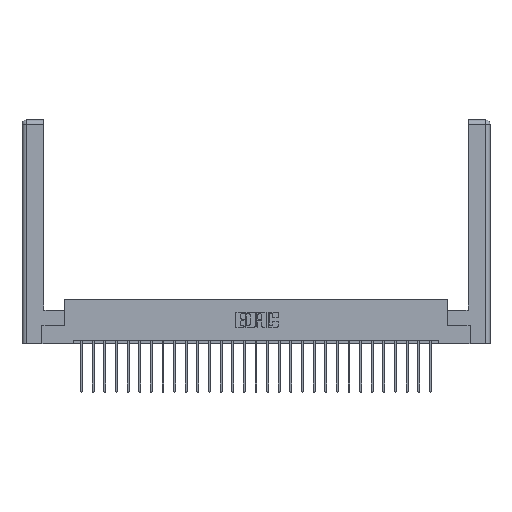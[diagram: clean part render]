
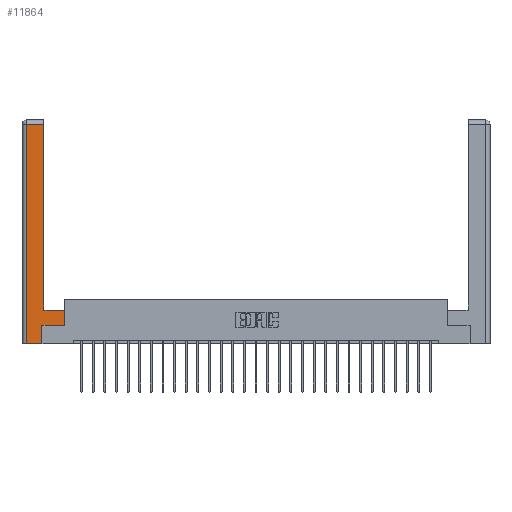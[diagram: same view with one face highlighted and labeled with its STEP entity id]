
A CAD part, top view. The second image highlights one B-rep face of the part: STEP entity #11864.
In plain terms, the highlighted planar face has unit normal (0, 0, 1).
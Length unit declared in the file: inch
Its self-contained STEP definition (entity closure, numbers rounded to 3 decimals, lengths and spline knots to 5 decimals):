
#12 = VERTEX_POINT ( 'NONE', #14965 ) ;
#310 = CARTESIAN_POINT ( 'NONE',  ( 0.565, 0.45, 0. ) ) ;
#606 = VERTEX_POINT ( 'NONE', #24938 ) ;
#802 = DIRECTION ( 'NONE',  ( 1., 0., 0. ) ) ;
#1749 = LINE ( 'NONE', #310, #18403 ) ;
#1751 = VERTEX_POINT ( 'NONE', #3683 ) ;
#1822 = VECTOR ( 'NONE', #13695, 39.37008 ) ;
#1941 = ORIENTED_EDGE ( 'NONE', *, *, #2260, .T. ) ;
#2144 = VECTOR ( 'NONE', #23206, 39.37008 ) ;
#2156 = VERTEX_POINT ( 'NONE', #4395 ) ;
#2260 = EDGE_CURVE ( 'NONE', #22480, #606, #15748, .T. ) ;
#2772 = CARTESIAN_POINT ( 'NONE',  ( 0.295, 0.45, 0. ) ) ;
#2914 = CARTESIAN_POINT ( 'NONE',  ( 0.0615, 2.94, 0. ) ) ;
#3683 = CARTESIAN_POINT ( 'NONE',  ( 0.265, 0.245, 0. ) ) ;
#3745 = CARTESIAN_POINT ( 'NONE',  ( 0.0615, 2.94, 0. ) ) ;
#4317 = ORIENTED_EDGE ( 'NONE', *, *, #19258, .T. ) ;
#4359 = VECTOR ( 'NONE', #12425, 39.37008 ) ;
#4395 = CARTESIAN_POINT ( 'NONE',  ( 0.295, 2.94, 0. ) ) ;
#4735 = ORIENTED_EDGE ( 'NONE', *, *, #16711, .T. ) ;
#4757 = ORIENTED_EDGE ( 'NONE', *, *, #23228, .T. ) ;
#4866 = AXIS2_PLACEMENT_3D ( 'NONE', #10646, #27982, #15006 ) ;
#5660 = CARTESIAN_POINT ( 'NONE',  ( 0.565, 0.245, 0. ) ) ;
#6412 = VECTOR ( 'NONE', #25604, 39.37008 ) ;
#7355 = VECTOR ( 'NONE', #26182, 39.37008 ) ;
#9174 = LINE ( 'NONE', #25433, #4359 ) ;
#9226 = VERTEX_POINT ( 'NONE', #2772 ) ;
#9634 = VECTOR ( 'NONE', #802, 39.37008 ) ;
#10209 = EDGE_LOOP ( 'NONE', ( #4317, #14536, #4735, #1941, #16208, #22615, #4757, #16655 ) ) ;
#10646 = CARTESIAN_POINT ( 'NONE',  ( 0., 0., 0. ) ) ;
#11552 = VECTOR ( 'NONE', #19246, 39.37008 ) ;
#11864 = ADVANCED_FACE ( 'NONE', ( #22489 ), #23612, .F. ) ;
#12425 = DIRECTION ( 'NONE',  ( -1., 0., 0. ) ) ;
#12521 = CARTESIAN_POINT ( 'NONE',  ( 0.565, 0.245, 0. ) ) ;
#13695 = DIRECTION ( 'NONE',  ( 0., -1., 0. ) ) ;
#14041 = LINE ( 'NONE', #2914, #2144 ) ;
#14451 = EDGE_CURVE ( 'NONE', #2156, #17685, #14041, .T. ) ;
#14536 = ORIENTED_EDGE ( 'NONE', *, *, #14451, .T. ) ;
#14965 = CARTESIAN_POINT ( 'NONE',  ( 0.565, 0.45, 0. ) ) ;
#15006 = DIRECTION ( 'NONE',  ( -1., 0., 0. ) ) ;
#15748 = LINE ( 'NONE', #26977, #9634 ) ;
#16208 = ORIENTED_EDGE ( 'NONE', *, *, #26216, .T. ) ;
#16595 = VERTEX_POINT ( 'NONE', #5660 ) ;
#16655 = ORIENTED_EDGE ( 'NONE', *, *, #19252, .T. ) ;
#16711 = EDGE_CURVE ( 'NONE', #17685, #22480, #25599, .T. ) ;
#17301 = CARTESIAN_POINT ( 'NONE',  ( 0.265, 0.245, 0. ) ) ;
#17685 = VERTEX_POINT ( 'NONE', #3745 ) ;
#18403 = VECTOR ( 'NONE', #26221, 39.37008 ) ;
#19246 = DIRECTION ( 'NONE',  ( 0., 1., 0. ) ) ;
#19252 = EDGE_CURVE ( 'NONE', #12, #9226, #9174, .T. ) ;
#19258 = EDGE_CURVE ( 'NONE', #9226, #2156, #26788, .T. ) ;
#19297 = EDGE_CURVE ( 'NONE', #1751, #16595, #21385, .T. ) ;
#20505 = CARTESIAN_POINT ( 'NONE',  ( 0.0615, 0., 0. ) ) ;
#21385 = LINE ( 'NONE', #12521, #6412 ) ;
#22480 = VERTEX_POINT ( 'NONE', #25348 ) ;
#22489 = FACE_OUTER_BOUND ( 'NONE', #10209, .T. ) ;
#22615 = ORIENTED_EDGE ( 'NONE', *, *, #19297, .T. ) ;
#23206 = DIRECTION ( 'NONE',  ( -1., 0., 0. ) ) ;
#23228 = EDGE_CURVE ( 'NONE', #16595, #12, #1749, .T. ) ;
#23612 = PLANE ( 'NONE',  #4866 ) ;
#23623 = LINE ( 'NONE', #17301, #7355 ) ;
#24938 = CARTESIAN_POINT ( 'NONE',  ( 0.265, 0., 0. ) ) ;
#25348 = CARTESIAN_POINT ( 'NONE',  ( 0.0615, 0., 0. ) ) ;
#25433 = CARTESIAN_POINT ( 'NONE',  ( 0.295, 0.45, 0. ) ) ;
#25599 = LINE ( 'NONE', #20505, #1822 ) ;
#25604 = DIRECTION ( 'NONE',  ( 1., 0., 0. ) ) ;
#25792 = CARTESIAN_POINT ( 'NONE',  ( 0.295, 3., 0. ) ) ;
#26182 = DIRECTION ( 'NONE',  ( 0., 1., 0. ) ) ;
#26216 = EDGE_CURVE ( 'NONE', #606, #1751, #23623, .T. ) ;
#26221 = DIRECTION ( 'NONE',  ( 0., 1., 0. ) ) ;
#26788 = LINE ( 'NONE', #25792, #11552 ) ;
#26977 = CARTESIAN_POINT ( 'NONE',  ( 0.265, 0., 0. ) ) ;
#27982 = DIRECTION ( 'NONE',  ( 0., 0., -1. ) ) ;
